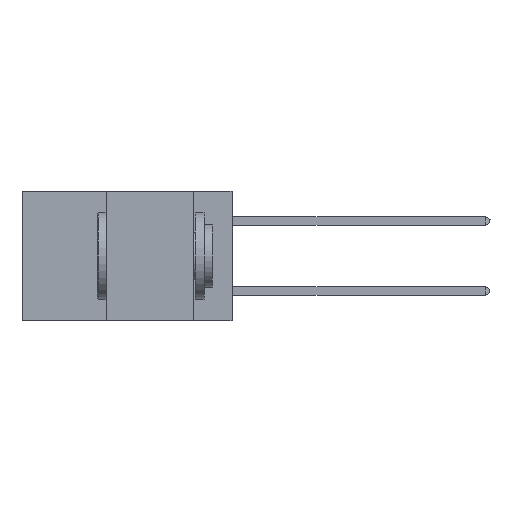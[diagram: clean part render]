
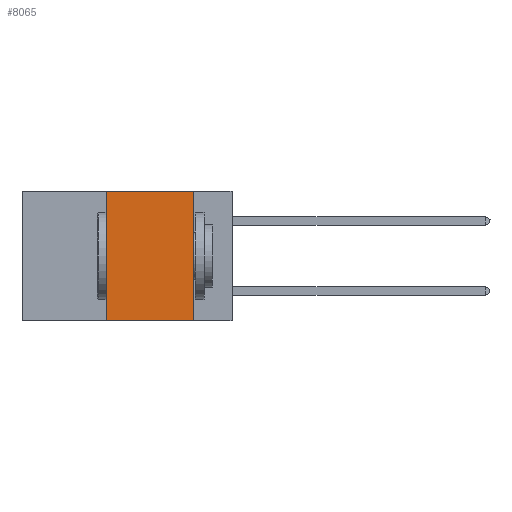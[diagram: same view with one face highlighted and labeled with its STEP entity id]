
A CAD part, left-side view. The second image highlights one B-rep face of the part: STEP entity #8065.
In plain terms, the highlighted planar face has unit normal (-1, 0, 0).
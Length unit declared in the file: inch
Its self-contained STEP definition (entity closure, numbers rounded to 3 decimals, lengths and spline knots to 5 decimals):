
#76 = ORIENTED_EDGE ( 'NONE', *, *, #13361, .T. ) ;
#763 = EDGE_CURVE ( 'NONE', #4148, #2894, #8690, .T. ) ;
#2005 = DIRECTION ( 'NONE',  ( 0., -1., 0. ) ) ;
#2755 = CARTESIAN_POINT ( 'NONE',  ( 0., 0.11, -0.37 ) ) ;
#2853 = FACE_OUTER_BOUND ( 'NONE', #4568, .T. ) ;
#2894 = VERTEX_POINT ( 'NONE', #9535 ) ;
#3438 = VERTEX_POINT ( 'NONE', #17664 ) ;
#3441 = LINE ( 'NONE', #17530, #6881 ) ;
#3481 = CARTESIAN_POINT ( 'NONE',  ( 0., 0.6, 0. ) ) ;
#4148 = VERTEX_POINT ( 'NONE', #4727 ) ;
#4224 = DIRECTION ( 'NONE',  ( 0., 0., -1. ) ) ;
#4568 = EDGE_LOOP ( 'NONE', ( #11103, #8786, #13602, #76 ) ) ;
#4727 = CARTESIAN_POINT ( 'NONE',  ( 0., 0.36, 0. ) ) ;
#4875 = CARTESIAN_POINT ( 'NONE',  ( 0., 0.36, 0. ) ) ;
#5787 = LINE ( 'NONE', #15794, #12652 ) ;
#6157 = VECTOR ( 'NONE', #14930, 39.37008 ) ;
#6496 = DIRECTION ( 'NONE',  ( 0., 0., 1. ) ) ;
#6828 = LINE ( 'NONE', #4875, #7967 ) ;
#6881 = VECTOR ( 'NONE', #2005, 39.37008 ) ;
#7967 = VECTOR ( 'NONE', #6496, 39.37008 ) ;
#8065 = ADVANCED_FACE ( 'NONE', ( #2853 ), #17979, .F. ) ;
#8690 = LINE ( 'NONE', #3481, #6157 ) ;
#8786 = ORIENTED_EDGE ( 'NONE', *, *, #763, .F. ) ;
#9535 = CARTESIAN_POINT ( 'NONE',  ( 0., 0.11, 0. ) ) ;
#10590 = AXIS2_PLACEMENT_3D ( 'NONE', #16520, #12255, #15131 ) ;
#11103 = ORIENTED_EDGE ( 'NONE', *, *, #17193, .F. ) ;
#11823 = EDGE_CURVE ( 'NONE', #3438, #4148, #6828, .T. ) ;
#12255 = DIRECTION ( 'NONE',  ( 1., 0., 0. ) ) ;
#12652 = VECTOR ( 'NONE', #4224, 39.37008 ) ;
#13361 = EDGE_CURVE ( 'NONE', #3438, #16757, #3441, .T. ) ;
#13602 = ORIENTED_EDGE ( 'NONE', *, *, #11823, .F. ) ;
#14930 = DIRECTION ( 'NONE',  ( 0., -1., 0. ) ) ;
#15131 = DIRECTION ( 'NONE',  ( 0., 0., -1. ) ) ;
#15794 = CARTESIAN_POINT ( 'NONE',  ( 0., 0.11, 0. ) ) ;
#16520 = CARTESIAN_POINT ( 'NONE',  ( 0., 0.6, 0. ) ) ;
#16757 = VERTEX_POINT ( 'NONE', #2755 ) ;
#17193 = EDGE_CURVE ( 'NONE', #2894, #16757, #5787, .T. ) ;
#17530 = CARTESIAN_POINT ( 'NONE',  ( 0., 0.6, -0.37 ) ) ;
#17664 = CARTESIAN_POINT ( 'NONE',  ( 0., 0.36, -0.37 ) ) ;
#17979 = PLANE ( 'NONE',  #10590 ) ;
